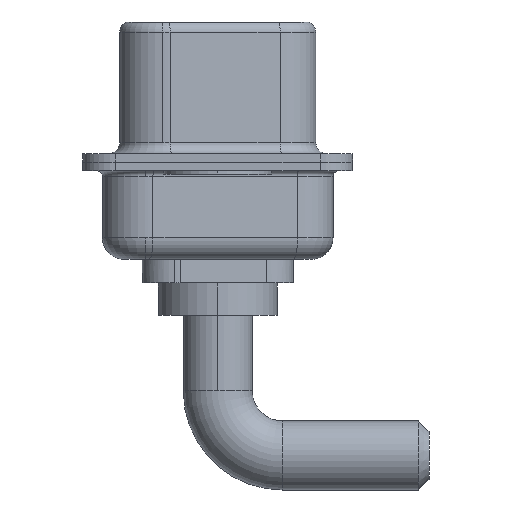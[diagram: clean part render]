
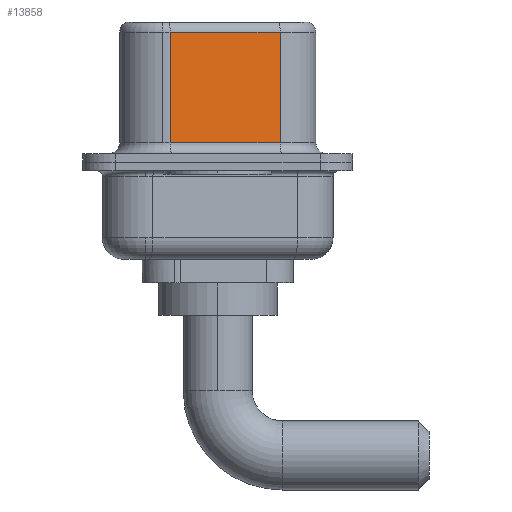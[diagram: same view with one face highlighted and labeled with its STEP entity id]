
A CAD part, left-side view. The second image highlights one B-rep face of the part: STEP entity #13858.
In plain terms, the highlighted planar face has unit normal (-0.985, -0.174, 0).
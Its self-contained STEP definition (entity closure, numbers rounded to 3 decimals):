
#97 = CARTESIAN_POINT ( 'NONE',  ( 3.655, 2.203, 6.02 ) ) ;
#220 = VECTOR ( 'NONE', #912, 1000. ) ;
#223 = EDGE_CURVE ( 'NONE', #5762, #11896, #3455, .T. ) ;
#424 = DIRECTION ( 'NONE',  ( -0.174, 0.985, 0. ) ) ;
#912 = DIRECTION ( 'NONE',  ( 0.174, -0.985, 0. ) ) ;
#1351 = CARTESIAN_POINT ( 'NONE',  ( 4.555, -2.897, 6.52 ) ) ;
#1395 = CARTESIAN_POINT ( 'NONE',  ( 4.555, -2.897, 6.02 ) ) ;
#1961 = LINE ( 'NONE', #10539, #220 ) ;
#2218 = LINE ( 'NONE', #6521, #5633 ) ;
#2346 = EDGE_CURVE ( 'NONE', #11356, #11896, #1961, .T. ) ;
#2401 = CARTESIAN_POINT ( 'NONE',  ( 4.555, -2.897, 6.52 ) ) ;
#2992 = AXIS2_PLACEMENT_3D ( 'NONE', #1351, #9860, #7707 ) ;
#3125 = VERTEX_POINT ( 'NONE', #97 ) ;
#3131 = CARTESIAN_POINT ( 'NONE',  ( 4.555, -2.897, 0.9 ) ) ;
#3455 = LINE ( 'NONE', #2401, #8225 ) ;
#5064 = EDGE_LOOP ( 'NONE', ( #5433, #13558, #10928, #10616 ) ) ;
#5433 = ORIENTED_EDGE ( 'NONE', *, *, #223, .F. ) ;
#5516 = FACE_OUTER_BOUND ( 'NONE', #5064, .T. ) ;
#5581 = PLANE ( 'NONE',  #2992 ) ;
#5633 = VECTOR ( 'NONE', #9811, 1000. ) ;
#5762 = VERTEX_POINT ( 'NONE', #10508 ) ;
#6521 = CARTESIAN_POINT ( 'NONE',  ( 3.655, 2.203, 6.52 ) ) ;
#7707 = DIRECTION ( 'NONE',  ( -0.174, 0.985, 0. ) ) ;
#8225 = VECTOR ( 'NONE', #10963, 1000. ) ;
#9811 = DIRECTION ( 'NONE',  ( 0., 0., -1. ) ) ;
#9838 = LINE ( 'NONE', #1395, #12358 ) ;
#9860 = DIRECTION ( 'NONE',  ( 0.985, 0.174, 0. ) ) ;
#9914 = EDGE_CURVE ( 'NONE', #3125, #11356, #2218, .T. ) ;
#9979 = EDGE_CURVE ( 'NONE', #5762, #3125, #9838, .T. ) ;
#10508 = CARTESIAN_POINT ( 'NONE',  ( 4.555, -2.897, 6.02 ) ) ;
#10539 = CARTESIAN_POINT ( 'NONE',  ( 4.555, -2.897, 0.9 ) ) ;
#10616 = ORIENTED_EDGE ( 'NONE', *, *, #2346, .T. ) ;
#10928 = ORIENTED_EDGE ( 'NONE', *, *, #9914, .T. ) ;
#10963 = DIRECTION ( 'NONE',  ( 0., 0., -1. ) ) ;
#11356 = VERTEX_POINT ( 'NONE', #12016 ) ;
#11896 = VERTEX_POINT ( 'NONE', #3131 ) ;
#12016 = CARTESIAN_POINT ( 'NONE',  ( 3.655, 2.203, 0.9 ) ) ;
#12358 = VECTOR ( 'NONE', #424, 1000. ) ;
#13558 = ORIENTED_EDGE ( 'NONE', *, *, #9979, .T. ) ;
#13858 = ADVANCED_FACE ( 'NONE', ( #5516 ), #5581, .F. ) ;
